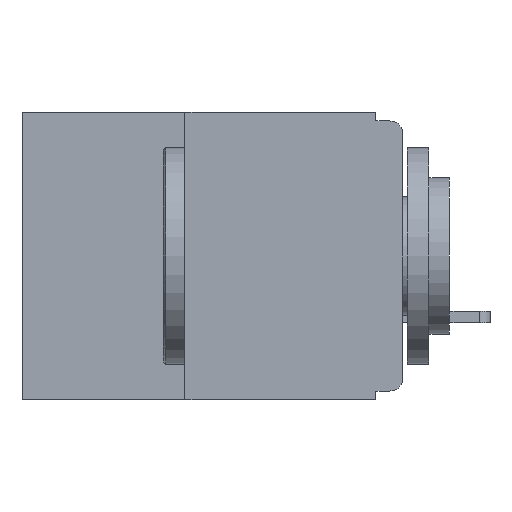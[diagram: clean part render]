
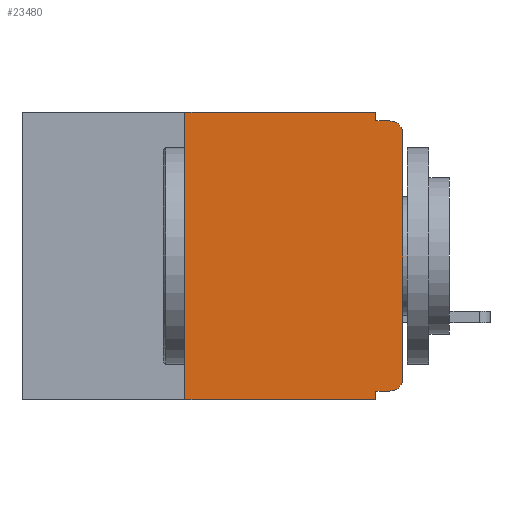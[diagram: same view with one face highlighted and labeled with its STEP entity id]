
A CAD part, left-side view. The second image highlights one B-rep face of the part: STEP entity #23480.
In plain terms, the highlighted planar face has unit normal (-1, 0, 0).
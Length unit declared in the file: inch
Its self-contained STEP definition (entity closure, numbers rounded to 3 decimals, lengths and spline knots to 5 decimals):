
#119 = VERTEX_POINT ( 'NONE', #14620 ) ;
#237 = EDGE_CURVE ( 'NONE', #1381, #119, #7995, .T. ) ;
#564 = VERTEX_POINT ( 'NONE', #9071 ) ;
#571 = ORIENTED_EDGE ( 'NONE', *, *, #237, .F. ) ;
#586 = DIRECTION ( 'NONE',  ( -1., 0., 0. ) ) ;
#1381 = VERTEX_POINT ( 'NONE', #22711 ) ;
#1530 = AXIS2_PLACEMENT_3D ( 'NONE', #11964, #586, #13843 ) ;
#1659 = LINE ( 'NONE', #4146, #21178 ) ;
#1742 = DIRECTION ( 'NONE',  ( 0., 1., 0. ) ) ;
#2288 = CARTESIAN_POINT ( 'NONE',  ( 0., 0.015, -0.32 ) ) ;
#2431 = VERTEX_POINT ( 'NONE', #10699 ) ;
#2434 = DIRECTION ( 'NONE',  ( 0., -1., 0. ) ) ;
#2546 = VECTOR ( 'NONE', #7355, 39.37008 ) ;
#3237 = EDGE_CURVE ( 'NONE', #23140, #12912, #5142, .T. ) ;
#3471 = ORIENTED_EDGE ( 'NONE', *, *, #7934, .T. ) ;
#4012 = CARTESIAN_POINT ( 'NONE',  ( 0., 0.031, -0.33 ) ) ;
#4143 = CARTESIAN_POINT ( 'NONE',  ( 0., 0., 0. ) ) ;
#4146 = CARTESIAN_POINT ( 'NONE',  ( 0., 0., -0.01 ) ) ;
#4595 = DIRECTION ( 'NONE',  ( 0., 0., 1. ) ) ;
#5142 = LINE ( 'NONE', #13402, #9641 ) ;
#5528 = DIRECTION ( 'NONE',  ( 0., -1., 0. ) ) ;
#5632 = AXIS2_PLACEMENT_3D ( 'NONE', #14616, #7060, #20292 ) ;
#6016 = EDGE_CURVE ( 'NONE', #564, #7737, #14544, .T. ) ;
#6085 = CARTESIAN_POINT ( 'NONE',  ( 0., 0.031, -0.32 ) ) ;
#6633 = VECTOR ( 'NONE', #13227, 39.37008 ) ;
#6677 = DIRECTION ( 'NONE',  ( -1., 0., 0. ) ) ;
#6755 = VECTOR ( 'NONE', #1742, 39.37008 ) ;
#6793 = ORIENTED_EDGE ( 'NONE', *, *, #8382, .F. ) ;
#6831 = VERTEX_POINT ( 'NONE', #6085 ) ;
#7060 = DIRECTION ( 'NONE',  ( 1., 0., 0. ) ) ;
#7347 = LINE ( 'NONE', #24312, #6755 ) ;
#7355 = DIRECTION ( 'NONE',  ( 0., 0., 1. ) ) ;
#7615 = LINE ( 'NONE', #18686, #2546 ) ;
#7702 = ORIENTED_EDGE ( 'NONE', *, *, #13428, .F. ) ;
#7737 = VERTEX_POINT ( 'NONE', #24400 ) ;
#7934 = EDGE_CURVE ( 'NONE', #7737, #2431, #11511, .T. ) ;
#7995 = LINE ( 'NONE', #20651, #17460 ) ;
#8382 = EDGE_CURVE ( 'NONE', #23140, #1381, #7615, .T. ) ;
#8924 = ORIENTED_EDGE ( 'NONE', *, *, #21455, .F. ) ;
#9071 = CARTESIAN_POINT ( 'NONE',  ( 0., 0., -0.305 ) ) ;
#9538 = VECTOR ( 'NONE', #4595, 39.37008 ) ;
#9641 = VECTOR ( 'NONE', #14081, 39.37008 ) ;
#10699 = CARTESIAN_POINT ( 'NONE',  ( 0., 0.015, -0.01 ) ) ;
#11350 = CARTESIAN_POINT ( 'NONE',  ( 0., 0.031, 0. ) ) ;
#11511 = CIRCLE ( 'NONE', #1530, 0.015 ) ;
#11572 = ORIENTED_EDGE ( 'NONE', *, *, #15405, .F. ) ;
#11964 = CARTESIAN_POINT ( 'NONE',  ( 0., 0.015, -0.025 ) ) ;
#12912 = VERTEX_POINT ( 'NONE', #4012 ) ;
#13004 = AXIS2_PLACEMENT_3D ( 'NONE', #18034, #6677, #19910 ) ;
#13061 = ORIENTED_EDGE ( 'NONE', *, *, #20554, .F. ) ;
#13227 = DIRECTION ( 'NONE',  ( 0., 0., -1. ) ) ;
#13402 = CARTESIAN_POINT ( 'NONE',  ( 0., 0.437, -0.33 ) ) ;
#13428 = EDGE_CURVE ( 'NONE', #119, #20433, #16708, .T. ) ;
#13715 = CARTESIAN_POINT ( 'NONE',  ( 0., 0.25, -0.33 ) ) ;
#13843 = DIRECTION ( 'NONE',  ( 0., 0., -1. ) ) ;
#14081 = DIRECTION ( 'NONE',  ( 0., -1., 0. ) ) ;
#14480 = ORIENTED_EDGE ( 'NONE', *, *, #6016, .T. ) ;
#14544 = LINE ( 'NONE', #4143, #9538 ) ;
#14616 = CARTESIAN_POINT ( 'NONE',  ( 0., 0.437, 0. ) ) ;
#14620 = CARTESIAN_POINT ( 'NONE',  ( 0., 0.031, 0. ) ) ;
#15231 = FACE_OUTER_BOUND ( 'NONE', #20668, .T. ) ;
#15405 = EDGE_CURVE ( 'NONE', #20433, #2431, #1659, .T. ) ;
#15433 = ORIENTED_EDGE ( 'NONE', *, *, #19791, .T. ) ;
#15768 = CARTESIAN_POINT ( 'NONE',  ( 0., 0.031, -0.33 ) ) ;
#16417 = CARTESIAN_POINT ( 'NONE',  ( 0., 0.031, -0.01 ) ) ;
#16708 = LINE ( 'NONE', #11350, #6633 ) ;
#17460 = VECTOR ( 'NONE', #5528, 39.37008 ) ;
#18034 = CARTESIAN_POINT ( 'NONE',  ( 0., 0.015, -0.305 ) ) ;
#18411 = PLANE ( 'NONE',  #5632 ) ;
#18581 = VECTOR ( 'NONE', #19554, 39.37008 ) ;
#18686 = CARTESIAN_POINT ( 'NONE',  ( 0., 0.25, -0.33 ) ) ;
#19554 = DIRECTION ( 'NONE',  ( 0., 0., -1. ) ) ;
#19574 = VERTEX_POINT ( 'NONE', #2288 ) ;
#19791 = EDGE_CURVE ( 'NONE', #19574, #564, #21862, .T. ) ;
#19826 = ORIENTED_EDGE ( 'NONE', *, *, #3237, .T. ) ;
#19910 = DIRECTION ( 'NONE',  ( 0., 0., -1. ) ) ;
#20292 = DIRECTION ( 'NONE',  ( 0., 0., -1. ) ) ;
#20433 = VERTEX_POINT ( 'NONE', #16417 ) ;
#20554 = EDGE_CURVE ( 'NONE', #19574, #6831, #7347, .T. ) ;
#20651 = CARTESIAN_POINT ( 'NONE',  ( 0., 0.437, 0. ) ) ;
#20668 = EDGE_LOOP ( 'NONE', ( #14480, #3471, #11572, #7702, #571, #6793, #19826, #8924, #13061, #15433 ) ) ;
#21178 = VECTOR ( 'NONE', #2434, 39.37008 ) ;
#21455 = EDGE_CURVE ( 'NONE', #6831, #12912, #24100, .T. ) ;
#21862 = CIRCLE ( 'NONE', #13004, 0.015 ) ;
#22711 = CARTESIAN_POINT ( 'NONE',  ( 0., 0.25, 0. ) ) ;
#23140 = VERTEX_POINT ( 'NONE', #13715 ) ;
#23480 = ADVANCED_FACE ( 'NONE', ( #15231 ), #18411, .F. ) ;
#24100 = LINE ( 'NONE', #15768, #18581 ) ;
#24312 = CARTESIAN_POINT ( 'NONE',  ( 0., 0., -0.32 ) ) ;
#24400 = CARTESIAN_POINT ( 'NONE',  ( 0., 0., -0.025 ) ) ;
